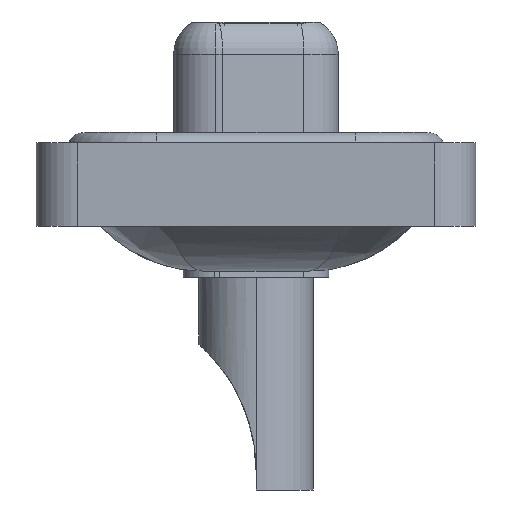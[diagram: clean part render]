
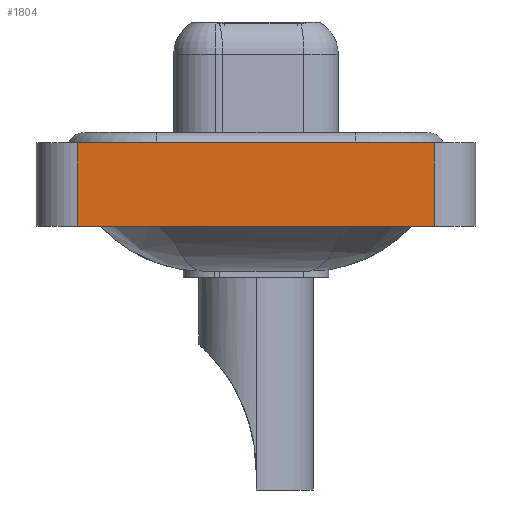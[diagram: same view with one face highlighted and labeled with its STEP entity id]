
A CAD part, left-side view. The second image highlights one B-rep face of the part: STEP entity #1804.
In plain terms, the highlighted planar face has unit normal (-1, 0, 0).
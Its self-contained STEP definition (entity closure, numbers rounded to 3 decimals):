
#685 = EDGE_LOOP ( 'NONE', ( #8666, #11890, #2051, #3997 ) ) ;
#858 = EDGE_CURVE ( 'NONE', #11463, #13184, #8534, .T. ) ;
#1804 = ADVANCED_FACE ( 'NONE', ( #8185 ), #8262, .T. ) ;
#1884 = DIRECTION ( 'NONE',  ( 0., -1., 0. ) ) ;
#2051 = ORIENTED_EDGE ( 'NONE', *, *, #858, .F. ) ;
#2995 = DIRECTION ( 'NONE',  ( 0., -1., 0. ) ) ;
#3206 = CARTESIAN_POINT ( 'NONE',  ( -7.25, -8.55, -3.6 ) ) ;
#3335 = DIRECTION ( 'NONE',  ( 0., 0., 1. ) ) ;
#3342 = LINE ( 'NONE', #8061, #13344 ) ;
#3648 = DIRECTION ( 'NONE',  ( 0., 0., 1. ) ) ;
#3997 = ORIENTED_EDGE ( 'NONE', *, *, #9384, .T. ) ;
#4577 = DIRECTION ( 'NONE',  ( -1., 0., 0. ) ) ;
#5883 = VERTEX_POINT ( 'NONE', #3206 ) ;
#8061 = CARTESIAN_POINT ( 'NONE',  ( -7.25, -8.55, 0.4 ) ) ;
#8185 = FACE_OUTER_BOUND ( 'NONE', #685, .T. ) ;
#8262 = PLANE ( 'NONE',  #12555 ) ;
#8534 = LINE ( 'NONE', #9503, #13167 ) ;
#8666 = ORIENTED_EDGE ( 'NONE', *, *, #13076, .T. ) ;
#9106 = VECTOR ( 'NONE', #3648, 1000. ) ;
#9164 = LINE ( 'NONE', #15262, #10346 ) ;
#9384 = EDGE_CURVE ( 'NONE', #11463, #5883, #9164, .T. ) ;
#9503 = CARTESIAN_POINT ( 'NONE',  ( -7.25, 8.55, -3.6 ) ) ;
#9816 = LINE ( 'NONE', #16082, #9106 ) ;
#10346 = VECTOR ( 'NONE', #2995, 1000. ) ;
#10518 = CARTESIAN_POINT ( 'NONE',  ( -7.25, -8.55, -3.6 ) ) ;
#11463 = VERTEX_POINT ( 'NONE', #14744 ) ;
#11890 = ORIENTED_EDGE ( 'NONE', *, *, #14428, .F. ) ;
#12188 = CARTESIAN_POINT ( 'NONE',  ( -7.25, 8.55, 0.4 ) ) ;
#12555 = AXIS2_PLACEMENT_3D ( 'NONE', #10518, #4577, #14259 ) ;
#13076 = EDGE_CURVE ( 'NONE', #5883, #14008, #9816, .T. ) ;
#13167 = VECTOR ( 'NONE', #3335, 1000. ) ;
#13184 = VERTEX_POINT ( 'NONE', #12188 ) ;
#13344 = VECTOR ( 'NONE', #1884, 1000. ) ;
#14008 = VERTEX_POINT ( 'NONE', #14803 ) ;
#14259 = DIRECTION ( 'NONE',  ( 0., 0., 1. ) ) ;
#14428 = EDGE_CURVE ( 'NONE', #13184, #14008, #3342, .T. ) ;
#14744 = CARTESIAN_POINT ( 'NONE',  ( -7.25, 8.55, -3.6 ) ) ;
#14803 = CARTESIAN_POINT ( 'NONE',  ( -7.25, -8.55, 0.4 ) ) ;
#15262 = CARTESIAN_POINT ( 'NONE',  ( -7.25, -8.55, -3.6 ) ) ;
#16082 = CARTESIAN_POINT ( 'NONE',  ( -7.25, -8.55, -3.6 ) ) ;
